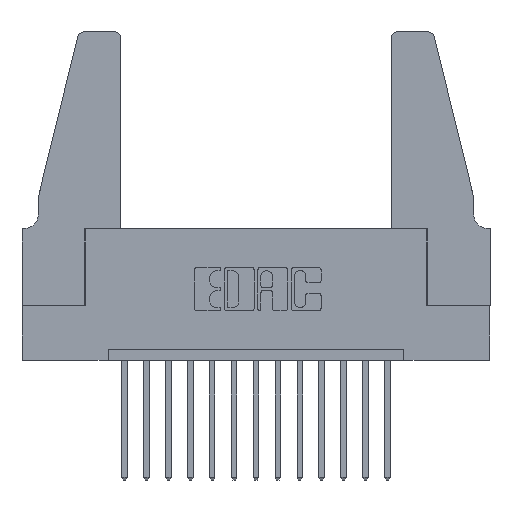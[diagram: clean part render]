
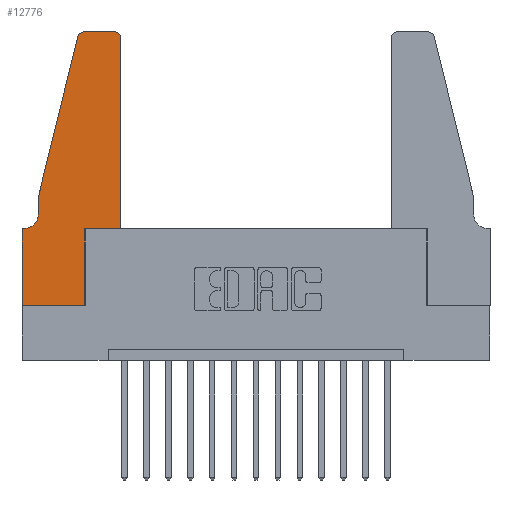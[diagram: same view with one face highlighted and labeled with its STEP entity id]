
A CAD part, top view. The second image highlights one B-rep face of the part: STEP entity #12776.
In plain terms, the highlighted planar face has unit normal (0, 0, 1).
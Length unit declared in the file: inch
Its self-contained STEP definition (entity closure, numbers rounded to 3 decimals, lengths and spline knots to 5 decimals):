
#71 = EDGE_CURVE ( 'NONE', #14011, #13712, #14960, .T. ) ;
#205 = CARTESIAN_POINT ( 'NONE',  ( 0.4505, 0.35, 0.37 ) ) ;
#460 = CARTESIAN_POINT ( 'NONE',  ( 0.2865, 0., 0.37 ) ) ;
#476 = DIRECTION ( 'NONE',  ( 1., 0., 0. ) ) ;
#542 = VERTEX_POINT ( 'NONE', #11510 ) ;
#694 = CARTESIAN_POINT ( 'NONE',  ( 0.4505, 0.35, 0.37 ) ) ;
#1021 = ORIENTED_EDGE ( 'NONE', *, *, #71, .T. ) ;
#1028 = VERTEX_POINT ( 'NONE', #14420 ) ;
#1101 = EDGE_CURVE ( 'NONE', #1028, #1765, #1184, .T. ) ;
#1176 = VECTOR ( 'NONE', #6513, 39.37008 ) ;
#1184 = CIRCLE ( 'NONE', #3449, 0.03 ) ;
#1234 = ORIENTED_EDGE ( 'NONE', *, *, #3906, .T. ) ;
#1442 = LINE ( 'NONE', #4868, #4849 ) ;
#1765 = VERTEX_POINT ( 'NONE', #3394 ) ;
#2530 = VECTOR ( 'NONE', #476, 39.37008 ) ;
#2609 = EDGE_CURVE ( 'NONE', #10708, #15752, #9130, .T. ) ;
#2630 = DIRECTION ( 'NONE',  ( 1., 0., 0. ) ) ;
#3259 = EDGE_CURVE ( 'NONE', #15752, #542, #12936, .T. ) ;
#3354 = AXIS2_PLACEMENT_3D ( 'NONE', #10578, #3369, #10625 ) ;
#3369 = DIRECTION ( 'NONE',  ( 0., 0., 1. ) ) ;
#3394 = CARTESIAN_POINT ( 'NONE',  ( 0.4205, 1.25, 0.37 ) ) ;
#3449 = AXIS2_PLACEMENT_3D ( 'NONE', #4758, #12160, #14681 ) ;
#3462 = LINE ( 'NONE', #13742, #1176 ) ;
#3809 = VECTOR ( 'NONE', #10312, 39.37008 ) ;
#3906 = EDGE_CURVE ( 'NONE', #13712, #15291, #8539, .T. ) ;
#4241 = FACE_OUTER_BOUND ( 'NONE', #7715, .T. ) ;
#4732 = EDGE_CURVE ( 'NONE', #11419, #9052, #13058, .T. ) ;
#4758 = CARTESIAN_POINT ( 'NONE',  ( 0.4205, 1.22, 0.37 ) ) ;
#4849 = VECTOR ( 'NONE', #12119, 39.37008 ) ;
#4868 = CARTESIAN_POINT ( 'NONE',  ( 0.0755, 0.35, 0.37 ) ) ;
#5152 = ORIENTED_EDGE ( 'NONE', *, *, #2609, .T. ) ;
#5157 = CARTESIAN_POINT ( 'NONE',  ( 0., 0., 0.37 ) ) ;
#5340 = EDGE_CURVE ( 'NONE', #542, #14815, #12211, .T. ) ;
#5581 = CARTESIAN_POINT ( 'NONE',  ( 0., 0.35, 0.37 ) ) ;
#5667 = VECTOR ( 'NONE', #11239, 39.37008 ) ;
#6030 = ORIENTED_EDGE ( 'NONE', *, *, #14587, .T. ) ;
#6513 = DIRECTION ( 'NONE',  ( -0.239, -0.971, 0. ) ) ;
#6826 = LINE ( 'NONE', #205, #7367 ) ;
#6870 = ORIENTED_EDGE ( 'NONE', *, *, #7140, .T. ) ;
#7140 = EDGE_CURVE ( 'NONE', #14815, #1028, #6826, .T. ) ;
#7367 = VECTOR ( 'NONE', #10097, 39.37008 ) ;
#7628 = ORIENTED_EDGE ( 'NONE', *, *, #9019, .T. ) ;
#7715 = EDGE_LOOP ( 'NONE', ( #6030, #14375, #13552, #1021, #1234, #12430, #7628, #5152, #13807, #11484, #6870, #11279 ) ) ;
#8427 = DIRECTION ( 'NONE',  ( 0., 0., 1. ) ) ;
#8539 = CIRCLE ( 'NONE', #9108, 0.07 ) ;
#8929 = CARTESIAN_POINT ( 'NONE',  ( 0.2865, 0.35, 0.37 ) ) ;
#9019 = EDGE_CURVE ( 'NONE', #10789, #10708, #12509, .T. ) ;
#9052 = VERTEX_POINT ( 'NONE', #9906 ) ;
#9104 = VECTOR ( 'NONE', #15670, 39.37008 ) ;
#9108 = AXIS2_PLACEMENT_3D ( 'NONE', #10175, #10226, #11300 ) ;
#9130 = LINE ( 'NONE', #12167, #11592 ) ;
#9432 = EDGE_CURVE ( 'NONE', #15291, #10789, #1442, .T. ) ;
#9796 = CARTESIAN_POINT ( 'NONE',  ( 0.284, 1.25, 0.37 ) ) ;
#9906 = CARTESIAN_POINT ( 'NONE',  ( 0.25487, 1.22718, 0.37 ) ) ;
#10097 = DIRECTION ( 'NONE',  ( 0., 1., 0. ) ) ;
#10175 = CARTESIAN_POINT ( 'NONE',  ( 0.0055, 0.42, 0.37 ) ) ;
#10226 = DIRECTION ( 'NONE',  ( 0., 0., -1. ) ) ;
#10312 = DIRECTION ( 'NONE',  ( -1., 0., 0. ) ) ;
#10578 = CARTESIAN_POINT ( 'NONE',  ( 0., 0.35, 0.37 ) ) ;
#10625 = DIRECTION ( 'NONE',  ( 1., 0., 0. ) ) ;
#10708 = VERTEX_POINT ( 'NONE', #5157 ) ;
#10789 = VERTEX_POINT ( 'NONE', #5581 ) ;
#10887 = LINE ( 'NONE', #15129, #3809 ) ;
#11239 = DIRECTION ( 'NONE',  ( 0., 1., 0. ) ) ;
#11259 = PLANE ( 'NONE',  #3354 ) ;
#11274 = VECTOR ( 'NONE', #11741, 39.37008 ) ;
#11279 = ORIENTED_EDGE ( 'NONE', *, *, #1101, .T. ) ;
#11300 = DIRECTION ( 'NONE',  ( -1., 0., 0. ) ) ;
#11419 = VERTEX_POINT ( 'NONE', #9796 ) ;
#11484 = ORIENTED_EDGE ( 'NONE', *, *, #5340, .T. ) ;
#11510 = CARTESIAN_POINT ( 'NONE',  ( 0.2865, 0.35, 0.37 ) ) ;
#11543 = CARTESIAN_POINT ( 'NONE',  ( 0.0755, 0.5, 0.37 ) ) ;
#11592 = VECTOR ( 'NONE', #14641, 39.37008 ) ;
#11741 = DIRECTION ( 'NONE',  ( 0., -1., 0. ) ) ;
#11966 = CARTESIAN_POINT ( 'NONE',  ( 0.0755, 0.42, 0.37 ) ) ;
#11984 = CARTESIAN_POINT ( 'NONE',  ( 0., 0., 0.37 ) ) ;
#12119 = DIRECTION ( 'NONE',  ( -1., 0., 0. ) ) ;
#12160 = DIRECTION ( 'NONE',  ( 0., 0., 1. ) ) ;
#12167 = CARTESIAN_POINT ( 'NONE',  ( 0., 0., 0.37 ) ) ;
#12211 = LINE ( 'NONE', #694, #2530 ) ;
#12430 = ORIENTED_EDGE ( 'NONE', *, *, #9432, .T. ) ;
#12509 = LINE ( 'NONE', #11984, #9104 ) ;
#12776 = ADVANCED_FACE ( 'NONE', ( #4241 ), #11259, .T. ) ;
#12936 = LINE ( 'NONE', #8929, #5667 ) ;
#13058 = CIRCLE ( 'NONE', #14031, 0.03 ) ;
#13176 = CARTESIAN_POINT ( 'NONE',  ( 0.0755, 0.5, 0.37 ) ) ;
#13552 = ORIENTED_EDGE ( 'NONE', *, *, #14422, .T. ) ;
#13712 = VERTEX_POINT ( 'NONE', #11966 ) ;
#13742 = CARTESIAN_POINT ( 'NONE',  ( 0.0755, 0.5, 0.37 ) ) ;
#13807 = ORIENTED_EDGE ( 'NONE', *, *, #3259, .T. ) ;
#14011 = VERTEX_POINT ( 'NONE', #13176 ) ;
#14031 = AXIS2_PLACEMENT_3D ( 'NONE', #15786, #8427, #2630 ) ;
#14375 = ORIENTED_EDGE ( 'NONE', *, *, #4732, .T. ) ;
#14420 = CARTESIAN_POINT ( 'NONE',  ( 0.4505, 1.22, 0.37 ) ) ;
#14422 = EDGE_CURVE ( 'NONE', #9052, #14011, #3462, .T. ) ;
#14587 = EDGE_CURVE ( 'NONE', #1765, #11419, #10887, .T. ) ;
#14641 = DIRECTION ( 'NONE',  ( 1., 0., 0. ) ) ;
#14681 = DIRECTION ( 'NONE',  ( 1., 0., 0. ) ) ;
#14690 = CARTESIAN_POINT ( 'NONE',  ( 0.4505, 0.35, 0.37 ) ) ;
#14815 = VERTEX_POINT ( 'NONE', #14690 ) ;
#14960 = LINE ( 'NONE', #11543, #11274 ) ;
#15129 = CARTESIAN_POINT ( 'NONE',  ( 0.2605, 1.25, 0.37 ) ) ;
#15291 = VERTEX_POINT ( 'NONE', #15355 ) ;
#15355 = CARTESIAN_POINT ( 'NONE',  ( 0.0055, 0.35, 0.37 ) ) ;
#15670 = DIRECTION ( 'NONE',  ( 0., -1., 0. ) ) ;
#15752 = VERTEX_POINT ( 'NONE', #460 ) ;
#15786 = CARTESIAN_POINT ( 'NONE',  ( 0.284, 1.22, 0.37 ) ) ;
